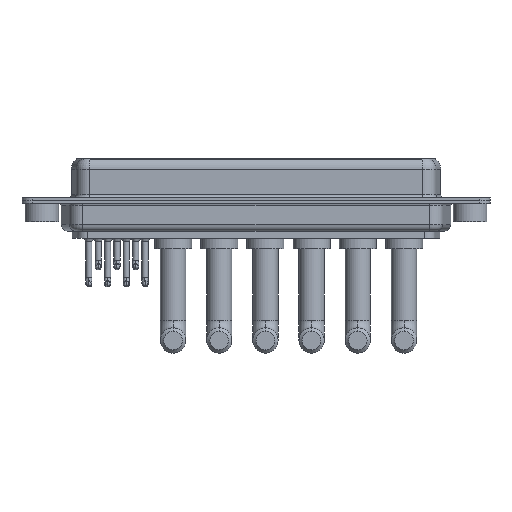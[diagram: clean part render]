
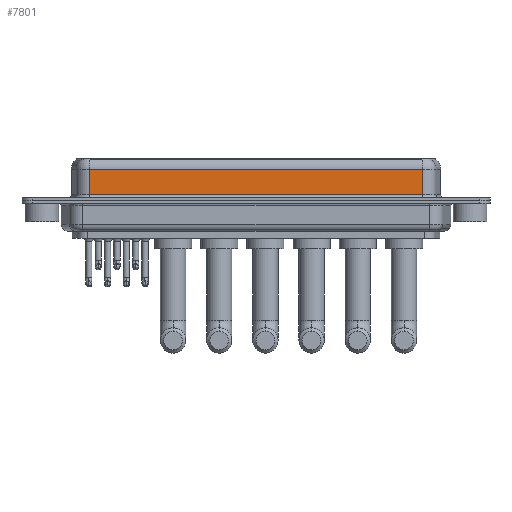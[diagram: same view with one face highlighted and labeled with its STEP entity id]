
A CAD part, front view. The second image highlights one B-rep face of the part: STEP entity #7801.
In plain terms, the highlighted planar face has unit normal (0, -1, 0).
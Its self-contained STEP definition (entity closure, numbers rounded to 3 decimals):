
#846 = VERTEX_POINT ( 'NONE', #12332 ) ;
#971 = ORIENTED_EDGE ( 'NONE', *, *, #7338, .T. ) ;
#1642 = DIRECTION ( 'NONE',  ( 0., 0., 1. ) ) ;
#2133 = ORIENTED_EDGE ( 'NONE', *, *, #5210, .T. ) ;
#2354 = VECTOR ( 'NONE', #7647, 1000. ) ;
#3052 = CARTESIAN_POINT ( 'NONE',  ( 56.462, -3.95, 0.9 ) ) ;
#3287 = VECTOR ( 'NONE', #7181, 1000. ) ;
#4165 = FACE_OUTER_BOUND ( 'NONE', #16345, .T. ) ;
#4514 = VERTEX_POINT ( 'NONE', #3052 ) ;
#5109 = LINE ( 'NONE', #6405, #2354 ) ;
#5210 = EDGE_CURVE ( 'NONE', #18053, #846, #5523, .T. ) ;
#5523 = LINE ( 'NONE', #15193, #16704 ) ;
#5744 = CARTESIAN_POINT ( 'NONE',  ( 56.462, -3.95, 6.4 ) ) ;
#6349 = ORIENTED_EDGE ( 'NONE', *, *, #16614, .T. ) ;
#6405 = CARTESIAN_POINT ( 'NONE',  ( 7.038, -3.95, 6.4 ) ) ;
#7067 = PLANE ( 'NONE',  #10819 ) ;
#7181 = DIRECTION ( 'NONE',  ( 0., 0., -1. ) ) ;
#7338 = EDGE_CURVE ( 'NONE', #846, #7631, #5109, .T. ) ;
#7631 = VERTEX_POINT ( 'NONE', #17092 ) ;
#7647 = DIRECTION ( 'NONE',  ( 0., 0., -1. ) ) ;
#7801 = ADVANCED_FACE ( 'NONE', ( #4165 ), #7067, .F. ) ;
#8672 = LINE ( 'NONE', #13148, #3287 ) ;
#8677 = VECTOR ( 'NONE', #9673, 1000. ) ;
#8741 = DIRECTION ( 'NONE',  ( 0., 1., 0. ) ) ;
#9249 = ORIENTED_EDGE ( 'NONE', *, *, #15826, .F. ) ;
#9673 = DIRECTION ( 'NONE',  ( 1., 0., 0. ) ) ;
#10819 = AXIS2_PLACEMENT_3D ( 'NONE', #5744, #8741, #1642 ) ;
#11025 = DIRECTION ( 'NONE',  ( -1., 0., 0. ) ) ;
#11694 = CARTESIAN_POINT ( 'NONE',  ( 56.462, -3.95, 4.65 ) ) ;
#12332 = CARTESIAN_POINT ( 'NONE',  ( 7.038, -3.95, 4.65 ) ) ;
#13148 = CARTESIAN_POINT ( 'NONE',  ( 56.462, -3.95, 6.4 ) ) ;
#13862 = CARTESIAN_POINT ( 'NONE',  ( 56.462, -3.95, 0.9 ) ) ;
#15193 = CARTESIAN_POINT ( 'NONE',  ( 56.462, -3.95, 4.65 ) ) ;
#15826 = EDGE_CURVE ( 'NONE', #18053, #4514, #8672, .T. ) ;
#16345 = EDGE_LOOP ( 'NONE', ( #9249, #2133, #971, #6349 ) ) ;
#16614 = EDGE_CURVE ( 'NONE', #7631, #4514, #16731, .T. ) ;
#16704 = VECTOR ( 'NONE', #11025, 1000. ) ;
#16731 = LINE ( 'NONE', #13862, #8677 ) ;
#17092 = CARTESIAN_POINT ( 'NONE',  ( 7.038, -3.95, 0.9 ) ) ;
#18053 = VERTEX_POINT ( 'NONE', #11694 ) ;
